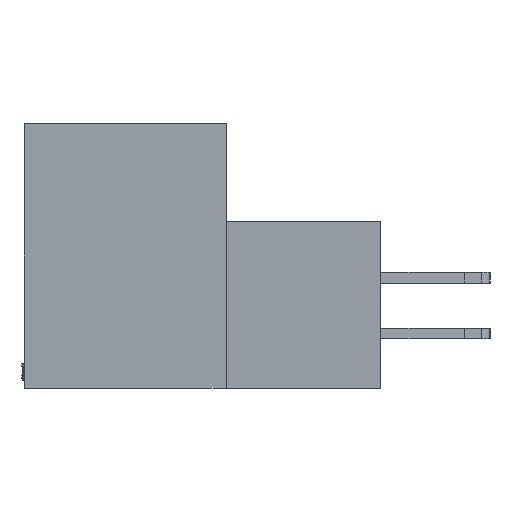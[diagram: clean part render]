
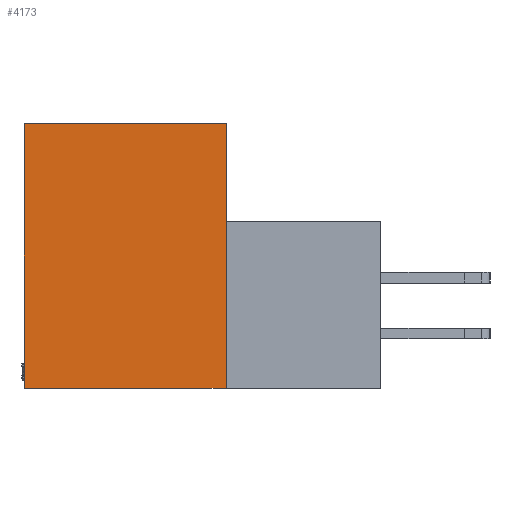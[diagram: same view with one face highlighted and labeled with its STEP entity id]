
A CAD part, left-side view. The second image highlights one B-rep face of the part: STEP entity #4173.
In plain terms, the highlighted planar face has unit normal (-1, 0, 0).
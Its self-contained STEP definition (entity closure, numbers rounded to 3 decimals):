
#520 = DIRECTION ( 'NONE',  ( 0., 0., 1. ) ) ;
#3611 = VECTOR ( 'NONE', #18609, 1000. ) ;
#3997 = EDGE_CURVE ( 'NONE', #8824, #24612, #17229, .T. ) ;
#4173 = ADVANCED_FACE ( 'NONE', ( #10494 ), #25769, .F. ) ;
#4216 = LINE ( 'NONE', #39638, #43270 ) ;
#6743 = AXIS2_PLACEMENT_3D ( 'NONE', #17284, #45091, #37280 ) ;
#8824 = VERTEX_POINT ( 'NONE', #35639 ) ;
#10494 = FACE_OUTER_BOUND ( 'NONE', #25358, .T. ) ;
#12624 = EDGE_CURVE ( 'NONE', #38349, #8824, #39436, .T. ) ;
#16063 = ORIENTED_EDGE ( 'NONE', *, *, #12624, .F. ) ;
#17229 = LINE ( 'NONE', #32745, #34615 ) ;
#17284 = CARTESIAN_POINT ( 'NONE',  ( 0., 0., 0. ) ) ;
#17602 = VERTEX_POINT ( 'NONE', #32365 ) ;
#18609 = DIRECTION ( 'NONE',  ( 0., -1., 0. ) ) ;
#24612 = VERTEX_POINT ( 'NONE', #26546 ) ;
#25358 = EDGE_LOOP ( 'NONE', ( #49270, #16063, #42837, #28757 ) ) ;
#25769 = PLANE ( 'NONE',  #6743 ) ;
#25881 = EDGE_CURVE ( 'NONE', #24612, #17602, #4216, .T. ) ;
#26546 = CARTESIAN_POINT ( 'NONE',  ( 0., 11.506, -15.088 ) ) ;
#27585 = VECTOR ( 'NONE', #29003, 1000. ) ;
#28757 = ORIENTED_EDGE ( 'NONE', *, *, #25881, .F. ) ;
#29003 = DIRECTION ( 'NONE',  ( 0., 0., -1. ) ) ;
#32229 = EDGE_CURVE ( 'NONE', #17602, #38349, #51338, .T. ) ;
#32365 = CARTESIAN_POINT ( 'NONE',  ( 0., 11.506, 0. ) ) ;
#32745 = CARTESIAN_POINT ( 'NONE',  ( 0., -8.814, -15.088 ) ) ;
#34615 = VECTOR ( 'NONE', #40917, 1000. ) ;
#35639 = CARTESIAN_POINT ( 'NONE',  ( 0., 0., -15.088 ) ) ;
#36189 = CARTESIAN_POINT ( 'NONE',  ( 0., 11.506, 0. ) ) ;
#37280 = DIRECTION ( 'NONE',  ( 0., 0., -1. ) ) ;
#38349 = VERTEX_POINT ( 'NONE', #49523 ) ;
#39436 = LINE ( 'NONE', #40491, #27585 ) ;
#39638 = CARTESIAN_POINT ( 'NONE',  ( 0., 11.506, -15.088 ) ) ;
#40491 = CARTESIAN_POINT ( 'NONE',  ( 0., 0., 0. ) ) ;
#40917 = DIRECTION ( 'NONE',  ( 0., 1., 0. ) ) ;
#42837 = ORIENTED_EDGE ( 'NONE', *, *, #32229, .F. ) ;
#43270 = VECTOR ( 'NONE', #520, 1000. ) ;
#45091 = DIRECTION ( 'NONE',  ( 1., 0., 0. ) ) ;
#49270 = ORIENTED_EDGE ( 'NONE', *, *, #3997, .F. ) ;
#49523 = CARTESIAN_POINT ( 'NONE',  ( 0., 0., 0. ) ) ;
#51338 = LINE ( 'NONE', #36189, #3611 ) ;
